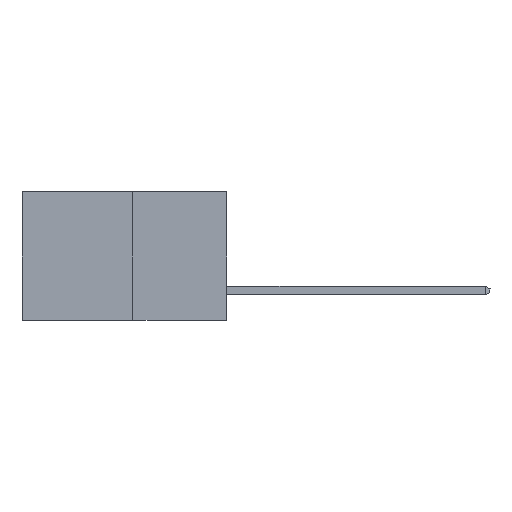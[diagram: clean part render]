
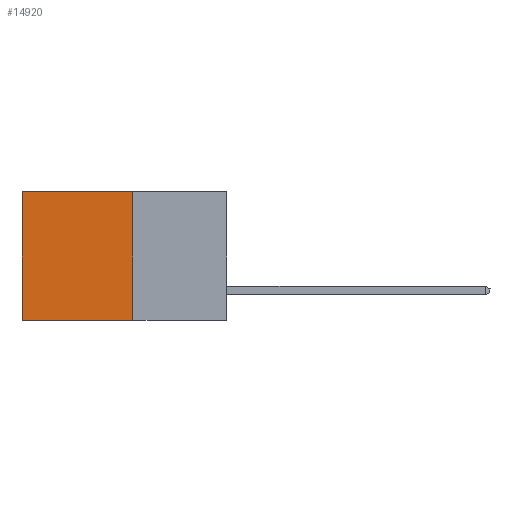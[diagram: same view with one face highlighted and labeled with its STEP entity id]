
A CAD part, left-side view. The second image highlights one B-rep face of the part: STEP entity #14920.
In plain terms, the highlighted planar face has unit normal (-1, 0, 0).
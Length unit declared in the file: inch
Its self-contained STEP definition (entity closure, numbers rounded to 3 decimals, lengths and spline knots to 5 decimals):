
#421 = LINE ( 'NONE', #5578, #4029 ) ;
#462 = LINE ( 'NONE', #9672, #12058 ) ;
#1075 = DIRECTION ( 'NONE',  ( 0., 0., -1. ) ) ;
#1525 = VERTEX_POINT ( 'NONE', #17332 ) ;
#2017 = VERTEX_POINT ( 'NONE', #8521 ) ;
#2198 = EDGE_CURVE ( 'NONE', #2017, #16398, #421, .T. ) ;
#2656 = DIRECTION ( 'NONE',  ( 0., 0., -1. ) ) ;
#3274 = AXIS2_PLACEMENT_3D ( 'NONE', #8697, #10173, #1075 ) ;
#4029 = VECTOR ( 'NONE', #2656, 39.37008 ) ;
#4236 = EDGE_LOOP ( 'NONE', ( #16892, #18554, #10398, #5049 ) ) ;
#5049 = ORIENTED_EDGE ( 'NONE', *, *, #10629, .T. ) ;
#5578 = CARTESIAN_POINT ( 'NONE',  ( 0.277, 0.59, -0.37 ) ) ;
#6466 = EDGE_CURVE ( 'NONE', #1525, #14156, #16696, .T. ) ;
#7524 = EDGE_CURVE ( 'NONE', #14156, #16398, #462, .T. ) ;
#8521 = CARTESIAN_POINT ( 'NONE',  ( 0.277, 0.59, 0. ) ) ;
#8618 = DIRECTION ( 'NONE',  ( 0., 0., -1. ) ) ;
#8697 = CARTESIAN_POINT ( 'NONE',  ( 0.277, 0.27, -0.37 ) ) ;
#9341 = CARTESIAN_POINT ( 'NONE',  ( 0.277, 0.59, -0.37 ) ) ;
#9672 = CARTESIAN_POINT ( 'NONE',  ( 0.277, 0.27, -0.37 ) ) ;
#10173 = DIRECTION ( 'NONE',  ( 1., 0., 0. ) ) ;
#10398 = ORIENTED_EDGE ( 'NONE', *, *, #6466, .F. ) ;
#10629 = EDGE_CURVE ( 'NONE', #1525, #2017, #14649, .T. ) ;
#11355 = CARTESIAN_POINT ( 'NONE',  ( 0.277, 0.27, -0.37 ) ) ;
#12058 = VECTOR ( 'NONE', #18442, 39.37008 ) ;
#12346 = VECTOR ( 'NONE', #8618, 39.37008 ) ;
#13721 = VECTOR ( 'NONE', #17418, 39.37008 ) ;
#14156 = VERTEX_POINT ( 'NONE', #11355 ) ;
#14649 = LINE ( 'NONE', #18867, #13721 ) ;
#14920 = ADVANCED_FACE ( 'NONE', ( #16264 ), #17498, .F. ) ;
#16264 = FACE_OUTER_BOUND ( 'NONE', #4236, .T. ) ;
#16398 = VERTEX_POINT ( 'NONE', #9341 ) ;
#16696 = LINE ( 'NONE', #17409, #12346 ) ;
#16892 = ORIENTED_EDGE ( 'NONE', *, *, #2198, .T. ) ;
#17332 = CARTESIAN_POINT ( 'NONE',  ( 0.277, 0.27, 0. ) ) ;
#17409 = CARTESIAN_POINT ( 'NONE',  ( 0.277, 0.27, -0.37 ) ) ;
#17418 = DIRECTION ( 'NONE',  ( 0., 1., 0. ) ) ;
#17498 = PLANE ( 'NONE',  #3274 ) ;
#18442 = DIRECTION ( 'NONE',  ( 0., 1., 0. ) ) ;
#18554 = ORIENTED_EDGE ( 'NONE', *, *, #7524, .F. ) ;
#18867 = CARTESIAN_POINT ( 'NONE',  ( 0.277, 0.27, 0. ) ) ;
